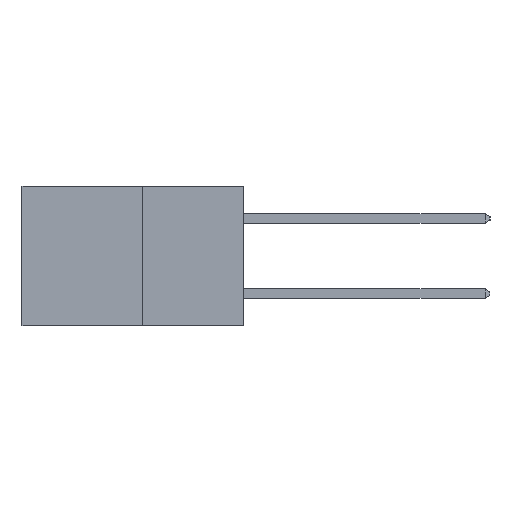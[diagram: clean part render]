
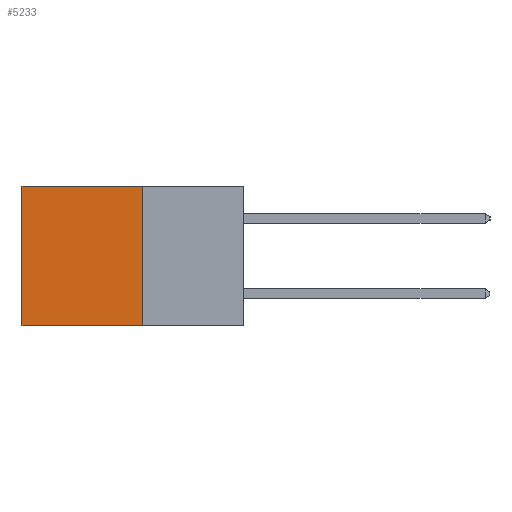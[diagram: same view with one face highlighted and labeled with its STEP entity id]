
A CAD part, left-side view. The second image highlights one B-rep face of the part: STEP entity #5233.
In plain terms, the highlighted planar face has unit normal (-1, 0, 0).
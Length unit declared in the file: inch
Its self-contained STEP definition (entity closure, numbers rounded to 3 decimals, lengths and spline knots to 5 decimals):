
#841 = EDGE_CURVE ( 'NONE', #20583, #11423, #9358, .T. ) ;
#862 = EDGE_CURVE ( 'NONE', #13490, #960, #7800, .T. ) ;
#960 = VERTEX_POINT ( 'NONE', #15331 ) ;
#1174 = VECTOR ( 'NONE', #13908, 39.37008 ) ;
#4004 = CARTESIAN_POINT ( 'NONE',  ( 0.277, 0.27, -0.37 ) ) ;
#4210 = CARTESIAN_POINT ( 'NONE',  ( 0.277, 0.27, 0. ) ) ;
#5233 = ADVANCED_FACE ( 'NONE', ( #17683 ), #27560, .F. ) ;
#5466 = EDGE_CURVE ( 'NONE', #960, #11423, #30930, .T. ) ;
#6667 = DIRECTION ( 'NONE',  ( 0., 1., 0. ) ) ;
#7800 = LINE ( 'NONE', #15723, #1174 ) ;
#9358 = LINE ( 'NONE', #9470, #20887 ) ;
#9470 = CARTESIAN_POINT ( 'NONE',  ( 0.277, 0.27, -0.37 ) ) ;
#10040 = CARTESIAN_POINT ( 'NONE',  ( 0.277, 0.27, -0.37 ) ) ;
#11423 = VERTEX_POINT ( 'NONE', #23736 ) ;
#11499 = DIRECTION ( 'NONE',  ( 0., 0., -1. ) ) ;
#12185 = AXIS2_PLACEMENT_3D ( 'NONE', #28091, #27498, #27457 ) ;
#12842 = ORIENTED_EDGE ( 'NONE', *, *, #18106, .F. ) ;
#12879 = VECTOR ( 'NONE', #11499, 39.37008 ) ;
#13490 = VERTEX_POINT ( 'NONE', #4210 ) ;
#13908 = DIRECTION ( 'NONE',  ( 0., 1., 0. ) ) ;
#15193 = ORIENTED_EDGE ( 'NONE', *, *, #5466, .T. ) ;
#15331 = CARTESIAN_POINT ( 'NONE',  ( 0.277, 0.59, 0. ) ) ;
#15723 = CARTESIAN_POINT ( 'NONE',  ( 0.277, 0.27, 0. ) ) ;
#15959 = EDGE_LOOP ( 'NONE', ( #15193, #27179, #12842, #16489 ) ) ;
#16489 = ORIENTED_EDGE ( 'NONE', *, *, #862, .T. ) ;
#17683 = FACE_OUTER_BOUND ( 'NONE', #15959, .T. ) ;
#18106 = EDGE_CURVE ( 'NONE', #13490, #20583, #19423, .T. ) ;
#19423 = LINE ( 'NONE', #4004, #12879 ) ;
#20583 = VERTEX_POINT ( 'NONE', #10040 ) ;
#20887 = VECTOR ( 'NONE', #6667, 39.37008 ) ;
#22261 = DIRECTION ( 'NONE',  ( 0., 0., -1. ) ) ;
#22472 = CARTESIAN_POINT ( 'NONE',  ( 0.277, 0.59, -0.37 ) ) ;
#23736 = CARTESIAN_POINT ( 'NONE',  ( 0.277, 0.59, -0.37 ) ) ;
#24563 = VECTOR ( 'NONE', #22261, 39.37008 ) ;
#27179 = ORIENTED_EDGE ( 'NONE', *, *, #841, .F. ) ;
#27457 = DIRECTION ( 'NONE',  ( 0., 0., -1. ) ) ;
#27498 = DIRECTION ( 'NONE',  ( 1., 0., 0. ) ) ;
#27560 = PLANE ( 'NONE',  #12185 ) ;
#28091 = CARTESIAN_POINT ( 'NONE',  ( 0.277, 0.27, -0.37 ) ) ;
#30930 = LINE ( 'NONE', #22472, #24563 ) ;
